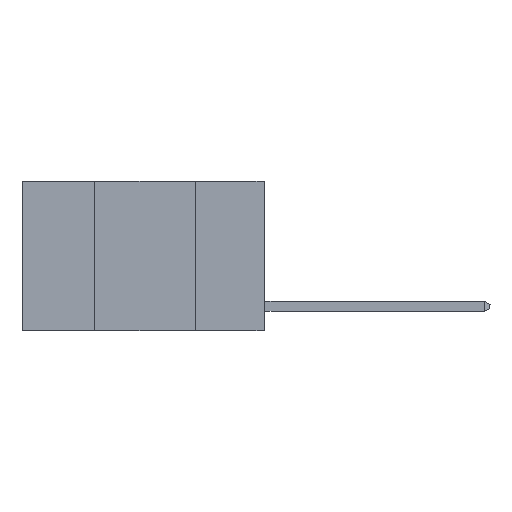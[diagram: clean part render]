
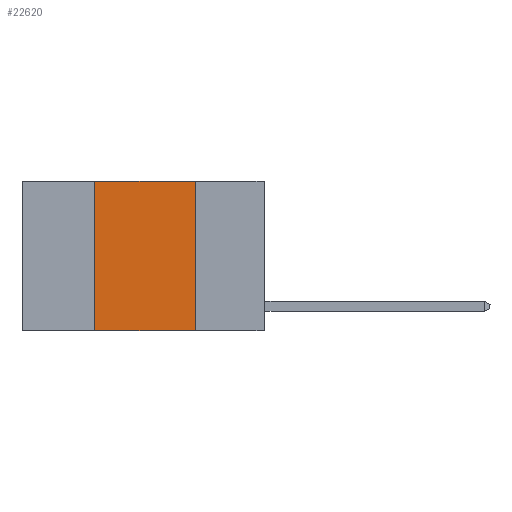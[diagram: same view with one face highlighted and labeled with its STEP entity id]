
A CAD part, left-side view. The second image highlights one B-rep face of the part: STEP entity #22620.
In plain terms, the highlighted planar face has unit normal (-1, 0, 0).
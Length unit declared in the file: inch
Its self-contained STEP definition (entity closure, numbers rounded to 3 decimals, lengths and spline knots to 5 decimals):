
#2172 = CARTESIAN_POINT ( 'NONE',  ( 0., 0.42, 0. ) ) ;
#2255 = ORIENTED_EDGE ( 'NONE', *, *, #24473, .F. ) ;
#2669 = VERTEX_POINT ( 'NONE', #27812 ) ;
#3673 = CARTESIAN_POINT ( 'NONE',  ( 0., 0.6, 0. ) ) ;
#4215 = VERTEX_POINT ( 'NONE', #23881 ) ;
#5315 = CARTESIAN_POINT ( 'NONE',  ( 0., 0.17, 0. ) ) ;
#6011 = DIRECTION ( 'NONE',  ( 1., 0., 0. ) ) ;
#6922 = VECTOR ( 'NONE', #20543, 39.37008 ) ;
#7280 = EDGE_CURVE ( 'NONE', #2669, #4215, #9622, .T. ) ;
#7370 = CARTESIAN_POINT ( 'NONE',  ( 0., 0.6, -0.37 ) ) ;
#7810 = EDGE_CURVE ( 'NONE', #15174, #4215, #19270, .T. ) ;
#8583 = VECTOR ( 'NONE', #23357, 39.37008 ) ;
#9622 = LINE ( 'NONE', #5315, #27106 ) ;
#10630 = FACE_OUTER_BOUND ( 'NONE', #19743, .T. ) ;
#13030 = LINE ( 'NONE', #2172, #6922 ) ;
#13084 = ORIENTED_EDGE ( 'NONE', *, *, #18004, .F. ) ;
#14533 = DIRECTION ( 'NONE',  ( 0., 0., -1. ) ) ;
#15174 = VERTEX_POINT ( 'NONE', #16299 ) ;
#15342 = CARTESIAN_POINT ( 'NONE',  ( 0., 0.42, 0. ) ) ;
#16299 = CARTESIAN_POINT ( 'NONE',  ( 0., 0.42, -0.37 ) ) ;
#17413 = PLANE ( 'NONE',  #23531 ) ;
#18004 = EDGE_CURVE ( 'NONE', #20654, #2669, #19557, .T. ) ;
#18114 = VECTOR ( 'NONE', #24626, 39.37008 ) ;
#19270 = LINE ( 'NONE', #7370, #8583 ) ;
#19557 = LINE ( 'NONE', #22340, #18114 ) ;
#19743 = EDGE_LOOP ( 'NONE', ( #24483, #13084, #2255, #20575 ) ) ;
#20543 = DIRECTION ( 'NONE',  ( 0., 0., 1. ) ) ;
#20575 = ORIENTED_EDGE ( 'NONE', *, *, #7810, .T. ) ;
#20654 = VERTEX_POINT ( 'NONE', #15342 ) ;
#21992 = DIRECTION ( 'NONE',  ( 0., 0., -1. ) ) ;
#22340 = CARTESIAN_POINT ( 'NONE',  ( 0., 0.6, 0. ) ) ;
#22620 = ADVANCED_FACE ( 'NONE', ( #10630 ), #17413, .F. ) ;
#23357 = DIRECTION ( 'NONE',  ( 0., -1., 0. ) ) ;
#23531 = AXIS2_PLACEMENT_3D ( 'NONE', #3673, #6011, #21992 ) ;
#23881 = CARTESIAN_POINT ( 'NONE',  ( 0., 0.17, -0.37 ) ) ;
#24473 = EDGE_CURVE ( 'NONE', #15174, #20654, #13030, .T. ) ;
#24483 = ORIENTED_EDGE ( 'NONE', *, *, #7280, .F. ) ;
#24626 = DIRECTION ( 'NONE',  ( 0., -1., 0. ) ) ;
#27106 = VECTOR ( 'NONE', #14533, 39.37008 ) ;
#27812 = CARTESIAN_POINT ( 'NONE',  ( 0., 0.17, 0. ) ) ;
